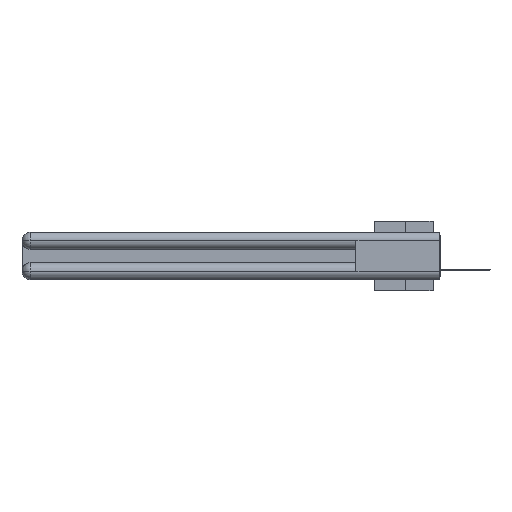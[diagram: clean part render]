
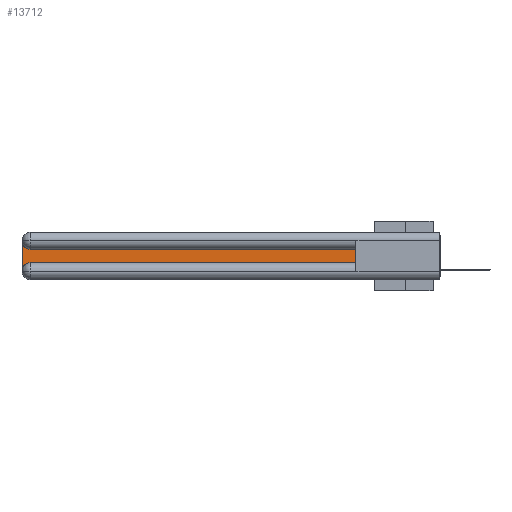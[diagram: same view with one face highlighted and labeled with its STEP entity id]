
A CAD part, left-side view. The second image highlights one B-rep face of the part: STEP entity #13712.
In plain terms, the highlighted planar face has unit normal (-1, 0, 0).
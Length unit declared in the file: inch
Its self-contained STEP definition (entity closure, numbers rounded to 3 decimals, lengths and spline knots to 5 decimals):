
#327 = EDGE_CURVE ( 'NONE', #21244, #3372, #23742, .T. ) ;
#345 = VERTEX_POINT ( 'NONE', #19475 ) ;
#430 = ORIENTED_EDGE ( 'NONE', *, *, #327, .T. ) ;
#1783 = EDGE_CURVE ( 'NONE', #345, #20495, #4003, .T. ) ;
#3246 = DIRECTION ( 'NONE',  ( 0., 0., -1. ) ) ;
#3370 = DIRECTION ( 'NONE',  ( 1., 0., 0. ) ) ;
#3372 = VERTEX_POINT ( 'NONE', #20765 ) ;
#4003 = LINE ( 'NONE', #31329, #24946 ) ;
#4317 = CIRCLE ( 'NONE', #22671, 0.06 ) ;
#4964 = VECTOR ( 'NONE', #13149, 39.37008 ) ;
#5998 = DIRECTION ( 'NONE',  ( 0., 0., 1. ) ) ;
#8556 = ORIENTED_EDGE ( 'NONE', *, *, #16810, .T. ) ;
#9335 = DIRECTION ( 'NONE',  ( 0., 0., -1. ) ) ;
#10499 = CARTESIAN_POINT ( 'NONE',  ( 0.075, 0.6, -0.2175 ) ) ;
#10820 = CARTESIAN_POINT ( 'NONE',  ( 0.075, 3., -0.1225 ) ) ;
#12481 = ORIENTED_EDGE ( 'NONE', *, *, #27137, .T. ) ;
#12641 = DIRECTION ( 'NONE',  ( 1., 0., 0. ) ) ;
#12667 = AXIS2_PLACEMENT_3D ( 'NONE', #10820, #3370, #3246 ) ;
#12975 = CARTESIAN_POINT ( 'NONE',  ( 0.075, 3., -0.0625 ) ) ;
#13149 = DIRECTION ( 'NONE',  ( 0., -1., 0. ) ) ;
#13712 = ADVANCED_FACE ( 'NONE', ( #17778 ), #16119, .F. ) ;
#13984 = CARTESIAN_POINT ( 'NONE',  ( 0.075, 0.6, -0.1225 ) ) ;
#16105 = EDGE_LOOP ( 'NONE', ( #31956, #27513, #430, #12481, #8556, #17332 ) ) ;
#16119 = PLANE ( 'NONE',  #12667 ) ;
#16513 = DIRECTION ( 'NONE',  ( 0., 1., 0. ) ) ;
#16713 = EDGE_CURVE ( 'NONE', #19705, #21244, #17997, .T. ) ;
#16810 = EDGE_CURVE ( 'NONE', #24598, #345, #18391, .T. ) ;
#17037 = VECTOR ( 'NONE', #9335, 39.37008 ) ;
#17332 = ORIENTED_EDGE ( 'NONE', *, *, #1783, .T. ) ;
#17778 = FACE_OUTER_BOUND ( 'NONE', #16105, .T. ) ;
#17997 = CIRCLE ( 'NONE', #25400, 0.06 ) ;
#18391 = LINE ( 'NONE', #10499, #4964 ) ;
#18749 = EDGE_CURVE ( 'NONE', #20495, #19705, #20226, .T. ) ;
#19475 = CARTESIAN_POINT ( 'NONE',  ( 0.075, 0.6, -0.2175 ) ) ;
#19705 = VERTEX_POINT ( 'NONE', #26606 ) ;
#20002 = CARTESIAN_POINT ( 'NONE',  ( 0.075, 2.94, -0.2775 ) ) ;
#20226 = LINE ( 'NONE', #13984, #21455 ) ;
#20495 = VERTEX_POINT ( 'NONE', #26727 ) ;
#20765 = CARTESIAN_POINT ( 'NONE',  ( 0.075, 3., -0.2775 ) ) ;
#21244 = VERTEX_POINT ( 'NONE', #12975 ) ;
#21249 = CARTESIAN_POINT ( 'NONE',  ( 0.075, 3., -0.2175 ) ) ;
#21455 = VECTOR ( 'NONE', #16513, 39.37008 ) ;
#22577 = DIRECTION ( 'NONE',  ( 0., 0., -1. ) ) ;
#22671 = AXIS2_PLACEMENT_3D ( 'NONE', #20002, #12641, #22577 ) ;
#22748 = DIRECTION ( 'NONE',  ( 0., 0., -1. ) ) ;
#23742 = LINE ( 'NONE', #21249, #17037 ) ;
#24455 = CARTESIAN_POINT ( 'NONE',  ( 0.075, 2.94, -0.2175 ) ) ;
#24598 = VERTEX_POINT ( 'NONE', #24455 ) ;
#24946 = VECTOR ( 'NONE', #5998, 39.37008 ) ;
#25400 = AXIS2_PLACEMENT_3D ( 'NONE', #29900, #32456, #22748 ) ;
#26606 = CARTESIAN_POINT ( 'NONE',  ( 0.075, 2.94, -0.1225 ) ) ;
#26727 = CARTESIAN_POINT ( 'NONE',  ( 0.075, 0.6, -0.1225 ) ) ;
#27137 = EDGE_CURVE ( 'NONE', #3372, #24598, #4317, .T. ) ;
#27513 = ORIENTED_EDGE ( 'NONE', *, *, #16713, .T. ) ;
#29900 = CARTESIAN_POINT ( 'NONE',  ( 0.075, 2.94, -0.0625 ) ) ;
#31329 = CARTESIAN_POINT ( 'NONE',  ( 0.075, 0.6, -0.2175 ) ) ;
#31956 = ORIENTED_EDGE ( 'NONE', *, *, #18749, .T. ) ;
#32456 = DIRECTION ( 'NONE',  ( 1., 0., 0. ) ) ;
